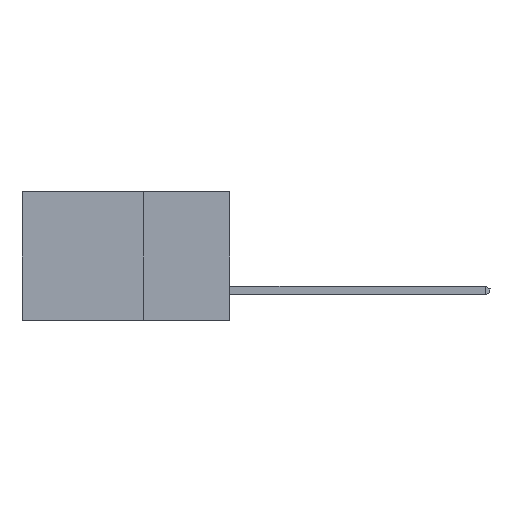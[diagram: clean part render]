
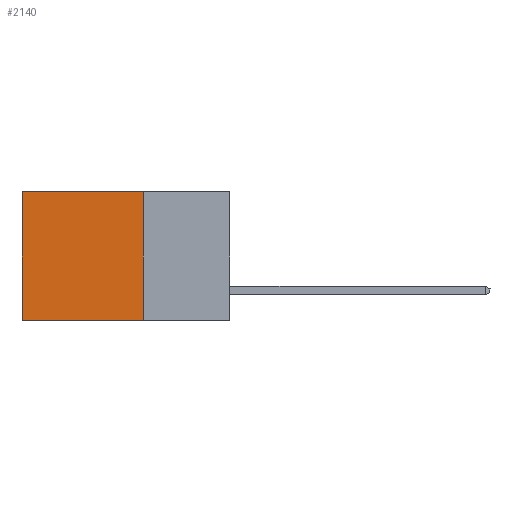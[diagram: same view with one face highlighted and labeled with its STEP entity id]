
A CAD part, left-side view. The second image highlights one B-rep face of the part: STEP entity #2140.
In plain terms, the highlighted planar face has unit normal (-1, 0, 0).
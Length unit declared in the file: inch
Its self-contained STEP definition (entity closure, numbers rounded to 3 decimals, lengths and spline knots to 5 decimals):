
#320 = PLANE ( 'NONE',  #6832 ) ;
#323 = DIRECTION ( 'NONE',  ( 0., 0., -1. ) ) ;
#390 = VECTOR ( 'NONE', #9804, 39.37008 ) ;
#556 = VERTEX_POINT ( 'NONE', #12878 ) ;
#865 = LINE ( 'NONE', #5405, #390 ) ;
#1091 = VECTOR ( 'NONE', #323, 39.37008 ) ;
#1632 = ORIENTED_EDGE ( 'NONE', *, *, #3433, .T. ) ;
#1653 = CARTESIAN_POINT ( 'NONE',  ( 0.2615, 0.25, -0.37 ) ) ;
#2049 = LINE ( 'NONE', #6573, #10126 ) ;
#2140 = ADVANCED_FACE ( 'NONE', ( #13018 ), #320, .F. ) ;
#2522 = LINE ( 'NONE', #8101, #11174 ) ;
#2777 = DIRECTION ( 'NONE',  ( 1., 0., 0. ) ) ;
#3212 = CARTESIAN_POINT ( 'NONE',  ( 0.2615, 0.6, 0. ) ) ;
#3433 = EDGE_CURVE ( 'NONE', #7108, #9321, #13020, .T. ) ;
#3948 = DIRECTION ( 'NONE',  ( 0., 0., -1. ) ) ;
#5187 = DIRECTION ( 'NONE',  ( 0., 1., 0. ) ) ;
#5405 = CARTESIAN_POINT ( 'NONE',  ( 0.2615, 0.25, -0.37 ) ) ;
#5793 = EDGE_CURVE ( 'NONE', #12139, #9321, #2049, .T. ) ;
#5944 = EDGE_CURVE ( 'NONE', #556, #12139, #865, .T. ) ;
#6573 = CARTESIAN_POINT ( 'NONE',  ( 0.2615, 0.25, -0.37 ) ) ;
#6832 = AXIS2_PLACEMENT_3D ( 'NONE', #1653, #2777, #3948 ) ;
#7108 = VERTEX_POINT ( 'NONE', #3212 ) ;
#8101 = CARTESIAN_POINT ( 'NONE',  ( 0.2615, 0.25, 0. ) ) ;
#8283 = EDGE_LOOP ( 'NONE', ( #1632, #9301, #9461, #14361 ) ) ;
#8335 = DIRECTION ( 'NONE',  ( 0., 1., 0. ) ) ;
#8510 = CARTESIAN_POINT ( 'NONE',  ( 0.2615, 0.25, -0.37 ) ) ;
#9301 = ORIENTED_EDGE ( 'NONE', *, *, #5793, .F. ) ;
#9321 = VERTEX_POINT ( 'NONE', #13493 ) ;
#9461 = ORIENTED_EDGE ( 'NONE', *, *, #5944, .F. ) ;
#9804 = DIRECTION ( 'NONE',  ( 0., 0., -1. ) ) ;
#10126 = VECTOR ( 'NONE', #5187, 39.37008 ) ;
#11174 = VECTOR ( 'NONE', #8335, 39.37008 ) ;
#11833 = CARTESIAN_POINT ( 'NONE',  ( 0.2615, 0.6, -0.37 ) ) ;
#12139 = VERTEX_POINT ( 'NONE', #8510 ) ;
#12577 = EDGE_CURVE ( 'NONE', #556, #7108, #2522, .T. ) ;
#12878 = CARTESIAN_POINT ( 'NONE',  ( 0.2615, 0.25, 0. ) ) ;
#13018 = FACE_OUTER_BOUND ( 'NONE', #8283, .T. ) ;
#13020 = LINE ( 'NONE', #11833, #1091 ) ;
#13493 = CARTESIAN_POINT ( 'NONE',  ( 0.2615, 0.6, -0.37 ) ) ;
#14361 = ORIENTED_EDGE ( 'NONE', *, *, #12577, .T. ) ;
